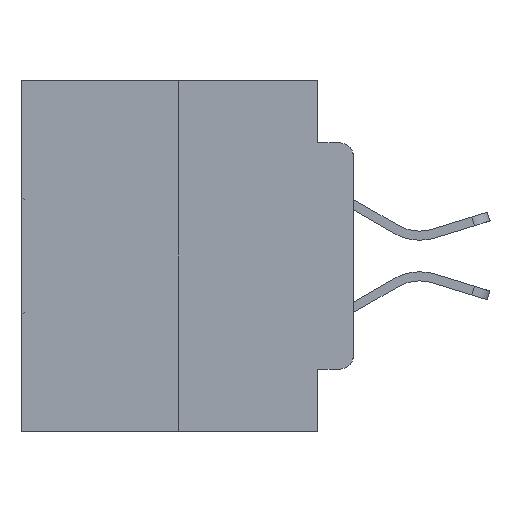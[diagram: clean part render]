
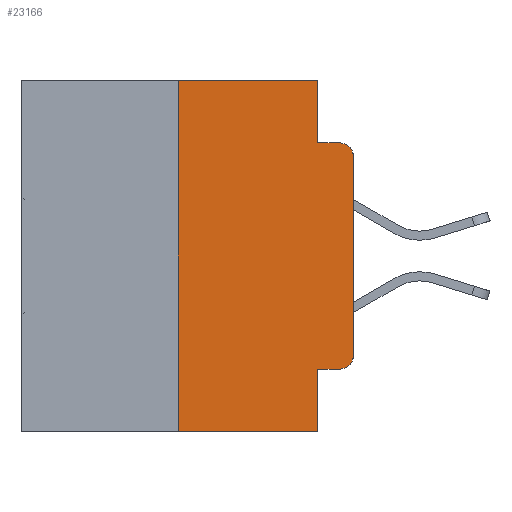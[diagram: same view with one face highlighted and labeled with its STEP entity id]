
A CAD part, left-side view. The second image highlights one B-rep face of the part: STEP entity #23166.
In plain terms, the highlighted planar face has unit normal (-1, 0, 0).
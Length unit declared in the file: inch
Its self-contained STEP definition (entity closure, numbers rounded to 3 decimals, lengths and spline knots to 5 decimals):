
#103 = VERTEX_POINT ( 'NONE', #17025 ) ;
#485 = DIRECTION ( 'NONE',  ( -1., 0., 0. ) ) ;
#1115 = ORIENTED_EDGE ( 'NONE', *, *, #18109, .F. ) ;
#1949 = VECTOR ( 'NONE', #8951, 39.37008 ) ;
#1991 = CARTESIAN_POINT ( 'NONE',  ( 0., 0.051, 0. ) ) ;
#2381 = VECTOR ( 'NONE', #16879, 39.37008 ) ;
#2441 = VECTOR ( 'NONE', #4032, 39.37008 ) ;
#2909 = LINE ( 'NONE', #22233, #26628 ) ;
#3817 = LINE ( 'NONE', #6292, #20757 ) ;
#4032 = DIRECTION ( 'NONE',  ( 0., -1., 0. ) ) ;
#4398 = LINE ( 'NONE', #7143, #26599 ) ;
#4715 = DIRECTION ( 'NONE',  ( 0., 0., 1. ) ) ;
#4777 = CARTESIAN_POINT ( 'NONE',  ( 0., 0.473, 0. ) ) ;
#5274 = ORIENTED_EDGE ( 'NONE', *, *, #22646, .T. ) ;
#5401 = CARTESIAN_POINT ( 'NONE',  ( 0., 0.051, 0. ) ) ;
#6292 = CARTESIAN_POINT ( 'NONE',  ( 0., 0.051, -0.0885 ) ) ;
#6515 = CARTESIAN_POINT ( 'NONE',  ( 0., 0.473, 0. ) ) ;
#7143 = CARTESIAN_POINT ( 'NONE',  ( 0., 0.25, 0. ) ) ;
#7206 = DIRECTION ( 'NONE',  ( 0., 0., -1. ) ) ;
#8951 = DIRECTION ( 'NONE',  ( 0., -1., 0. ) ) ;
#9033 = EDGE_CURVE ( 'NONE', #18527, #11662, #19976, .T. ) ;
#9416 = EDGE_CURVE ( 'NONE', #18585, #18009, #22761, .T. ) ;
#9937 = VERTEX_POINT ( 'NONE', #19692 ) ;
#10370 = LINE ( 'NONE', #29073, #2441 ) ;
#10579 = EDGE_CURVE ( 'NONE', #9937, #18527, #10370, .T. ) ;
#11000 = LINE ( 'NONE', #26551, #16971 ) ;
#11454 = CARTESIAN_POINT ( 'NONE',  ( 0., 0.051, -0.5 ) ) ;
#11662 = VERTEX_POINT ( 'NONE', #17131 ) ;
#11800 = PLANE ( 'NONE',  #13453 ) ;
#12160 = CARTESIAN_POINT ( 'NONE',  ( 0., 0.02, -0.3915 ) ) ;
#13453 = AXIS2_PLACEMENT_3D ( 'NONE', #4777, #20853, #7206 ) ;
#13503 = CARTESIAN_POINT ( 'NONE',  ( 0., 0.051, -0.0885 ) ) ;
#14210 = LINE ( 'NONE', #5401, #2381 ) ;
#14452 = DIRECTION ( 'NONE',  ( 0., 0., -1. ) ) ;
#14503 = LINE ( 'NONE', #6515, #1949 ) ;
#14629 = CARTESIAN_POINT ( 'NONE',  ( 0., 0.02, -0.1085 ) ) ;
#15769 = VERTEX_POINT ( 'NONE', #27548 ) ;
#16364 = VERTEX_POINT ( 'NONE', #1991 ) ;
#16422 = FACE_OUTER_BOUND ( 'NONE', #26834, .T. ) ;
#16498 = ORIENTED_EDGE ( 'NONE', *, *, #10579, .T. ) ;
#16609 = EDGE_CURVE ( 'NONE', #9937, #18009, #14210, .T. ) ;
#16837 = DIRECTION ( 'NONE',  ( 0., 0., -1. ) ) ;
#16879 = DIRECTION ( 'NONE',  ( 0., 0., -1. ) ) ;
#16971 = VECTOR ( 'NONE', #22022, 39.37008 ) ;
#17025 = CARTESIAN_POINT ( 'NONE',  ( 0., 0.25, 0. ) ) ;
#17131 = CARTESIAN_POINT ( 'NONE',  ( 0., 0., -0.3915 ) ) ;
#17278 = AXIS2_PLACEMENT_3D ( 'NONE', #12160, #27894, #14452 ) ;
#17536 = ORIENTED_EDGE ( 'NONE', *, *, #21122, .F. ) ;
#18009 = VERTEX_POINT ( 'NONE', #11454 ) ;
#18109 = EDGE_CURVE ( 'NONE', #18585, #103, #4398, .T. ) ;
#18527 = VERTEX_POINT ( 'NONE', #20103 ) ;
#18585 = VERTEX_POINT ( 'NONE', #24824 ) ;
#18936 = ORIENTED_EDGE ( 'NONE', *, *, #20404, .F. ) ;
#19629 = EDGE_CURVE ( 'NONE', #16364, #26133, #11000, .T. ) ;
#19692 = CARTESIAN_POINT ( 'NONE',  ( 0., 0.051, -0.4115 ) ) ;
#19976 = CIRCLE ( 'NONE', #17278, 0.02 ) ;
#20025 = DIRECTION ( 'NONE',  ( 0., -1., 0. ) ) ;
#20103 = CARTESIAN_POINT ( 'NONE',  ( 0., 0.02, -0.4115 ) ) ;
#20188 = DIRECTION ( 'NONE',  ( 0., -1., 0. ) ) ;
#20404 = EDGE_CURVE ( 'NONE', #103, #16364, #14503, .T. ) ;
#20542 = VERTEX_POINT ( 'NONE', #29508 ) ;
#20757 = VECTOR ( 'NONE', #20188, 39.37008 ) ;
#20853 = DIRECTION ( 'NONE',  ( 1., 0., 0. ) ) ;
#21122 = EDGE_CURVE ( 'NONE', #26133, #15769, #3817, .T. ) ;
#21340 = VECTOR ( 'NONE', #20025, 39.37008 ) ;
#22022 = DIRECTION ( 'NONE',  ( 0., 0., -1. ) ) ;
#22127 = ORIENTED_EDGE ( 'NONE', *, *, #24170, .T. ) ;
#22233 = CARTESIAN_POINT ( 'NONE',  ( 0., 0., 0. ) ) ;
#22402 = CARTESIAN_POINT ( 'NONE',  ( 0., 0.473, -0.5 ) ) ;
#22646 = EDGE_CURVE ( 'NONE', #20542, #15769, #23857, .T. ) ;
#22761 = LINE ( 'NONE', #22402, #21340 ) ;
#23166 = ADVANCED_FACE ( 'NONE', ( #16422 ), #11800, .F. ) ;
#23178 = ORIENTED_EDGE ( 'NONE', *, *, #9033, .T. ) ;
#23573 = AXIS2_PLACEMENT_3D ( 'NONE', #14629, #485, #16837 ) ;
#23857 = CIRCLE ( 'NONE', #23573, 0.02 ) ;
#24170 = EDGE_CURVE ( 'NONE', #11662, #20542, #2909, .T. ) ;
#24824 = CARTESIAN_POINT ( 'NONE',  ( 0., 0.25, -0.5 ) ) ;
#26133 = VERTEX_POINT ( 'NONE', #13503 ) ;
#26363 = ORIENTED_EDGE ( 'NONE', *, *, #9416, .T. ) ;
#26551 = CARTESIAN_POINT ( 'NONE',  ( 0., 0.051, 0. ) ) ;
#26599 = VECTOR ( 'NONE', #4715, 39.37008 ) ;
#26628 = VECTOR ( 'NONE', #28973, 39.37008 ) ;
#26834 = EDGE_LOOP ( 'NONE', ( #22127, #5274, #17536, #29457, #18936, #1115, #26363, #27745, #16498, #23178 ) ) ;
#27548 = CARTESIAN_POINT ( 'NONE',  ( 0., 0.02, -0.0885 ) ) ;
#27745 = ORIENTED_EDGE ( 'NONE', *, *, #16609, .F. ) ;
#27894 = DIRECTION ( 'NONE',  ( -1., 0., 0. ) ) ;
#28973 = DIRECTION ( 'NONE',  ( 0., 0., 1. ) ) ;
#29073 = CARTESIAN_POINT ( 'NONE',  ( 0., 0.051, -0.4115 ) ) ;
#29457 = ORIENTED_EDGE ( 'NONE', *, *, #19629, .F. ) ;
#29508 = CARTESIAN_POINT ( 'NONE',  ( 0., 0., -0.1085 ) ) ;
